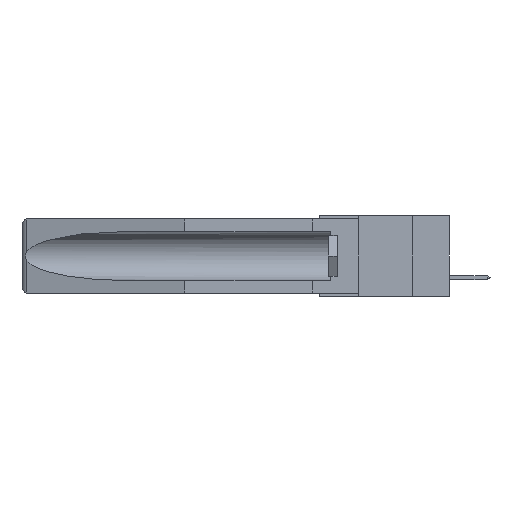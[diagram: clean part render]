
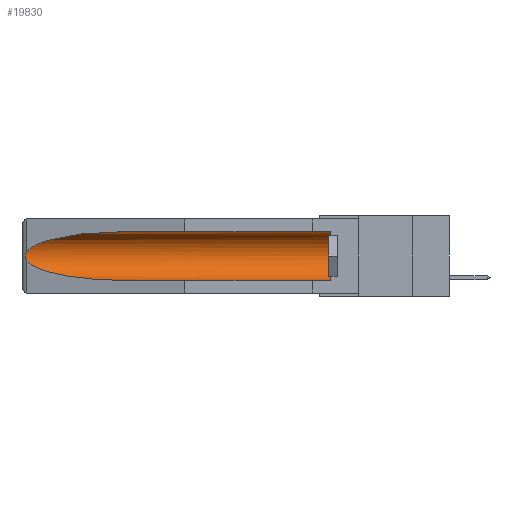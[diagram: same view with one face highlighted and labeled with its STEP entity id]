
A CAD part, left-side view. The second image highlights one B-rep face of the part: STEP entity #19830.
In plain terms, the highlighted cylindrical face has radius 2.857 mm (diameter 5.715 mm), a partial arc.
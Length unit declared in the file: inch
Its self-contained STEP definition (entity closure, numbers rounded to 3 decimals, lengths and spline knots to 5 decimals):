
#290 = EDGE_CURVE ( 'NONE', #24988, #15728, #14196, .T. ) ;
#362 = CARTESIAN_POINT ( 'NONE',  ( 0.155, 1.07973, -0.284 ) ) ;
#722 = ORIENTED_EDGE ( 'NONE', *, *, #5472, .T. ) ;
#1000 = ORIENTED_EDGE ( 'NONE', *, *, #20695, .T. ) ;
#1009 = CARTESIAN_POINT ( 'NONE',  ( 0.2675, 1.53308, -0.17534 ) ) ;
#1098 = CYLINDRICAL_SURFACE ( 'NONE', #19582, 0.1125 ) ;
#1209 = CARTESIAN_POINT ( 'NONE',  ( 0.26654, 1.53092, -0.15636 ) ) ;
#1514 = DIRECTION ( 'NONE',  ( 0., 1., 0. ) ) ;
#1770 = CARTESIAN_POINT ( 'NONE',  ( 0.25451, 1.48313, -0.09465 ) ) ;
#1946 = DIRECTION ( 'NONE',  ( 0., 0., 1. ) ) ;
#2255 = CARTESIAN_POINT ( 'NONE',  ( 0.25451, 1.48313, -0.24835 ) ) ;
#3594 = ORIENTED_EDGE ( 'NONE', *, *, #12901, .T. ) ;
#5472 = EDGE_CURVE ( 'NONE', #19635, #10450, #25865, .T. ) ;
#5909 = CARTESIAN_POINT ( 'NONE',  ( 0.2673, 1.53269, -0.17917 ) ) ;
#6745 = CARTESIAN_POINT ( 'NONE',  ( 0.26537, 1.52718, -0.19328 ) ) ;
#7039 = CARTESIAN_POINT ( 'NONE',  ( 0.26597, 1.5296, -0.19026 ) ) ;
#7882 = CARTESIAN_POINT ( 'NONE',  ( 0.155, 0.126, -0.1715 ) ) ;
#8403 = DIRECTION ( 'NONE',  ( 0., 0., 1. ) ) ;
#8800 = ORIENTED_EDGE ( 'NONE', *, *, #290, .T. ) ;
#8881 = VECTOR ( 'NONE', #13621, 39.37008 ) ;
#9677 = CARTESIAN_POINT ( 'NONE',  ( 0.21114, 1.30732, -0.284 ) ) ;
#10450 = VERTEX_POINT ( 'NONE', #31261 ) ;
#10668 = CARTESIAN_POINT ( 'NONE',  ( 0.2675, 1.53308, -0.16763 ) ) ;
#11177 = CARTESIAN_POINT ( 'NONE',  ( 0.155, -0.30754, -0.059 ) ) ;
#11340 = FACE_OUTER_BOUND ( 'NONE', #30940, .T. ) ;
#11903 = LINE ( 'NONE', #11177, #8881 ) ;
#12901 = EDGE_CURVE ( 'NONE', #15728, #19635, #11903, .T. ) ;
#13092 = CARTESIAN_POINT ( 'NONE',  ( 0.2673, 1.5327, -0.16383 ) ) ;
#13621 = DIRECTION ( 'NONE',  ( 0., 1., 0. ) ) ;
#13693 = ORIENTED_EDGE ( 'NONE', *, *, #15148, .F. ) ;
#13816 = B_SPLINE_CURVE_WITH_KNOTS ( 'NONE', 3,
 ( #25207, #15742, #1209, #13092, #10668, #1009, #5909, #31341, #7039, #6745 ),
 .UNSPECIFIED., .F., .F.,
 ( 4, 2, 2, 2, 4 ),
 ( 0., 0.00029, 0.00058, 0.00087, 0.00117 ),
 .UNSPECIFIED. ) ;
#13850 = CARTESIAN_POINT ( 'NONE',  ( 0.21114, 1.30732, -0.059 ) ) ;
#14196 = CIRCLE ( 'NONE', #25881, 0.1125 ) ;
#14233 = CARTESIAN_POINT ( 'NONE',  ( 0.155, -0.30754, -0.1715 ) ) ;
#14399 =( BOUNDED_CURVE ( )  B_SPLINE_CURVE ( 3, ( #31339, #2255, #9677, #31130 ),
 .UNSPECIFIED., .F., .F. ) 
 B_SPLINE_CURVE_WITH_KNOTS ( ( 4, 4 ),
 ( 0.1948, 1.5708 ),
 .UNSPECIFIED. ) 
 CURVE ( )  GEOMETRIC_REPRESENTATION_ITEM ( )  RATIONAL_B_SPLINE_CURVE ( ( 1., 0.848, 0.848, 1. ) ) 
 REPRESENTATION_ITEM ( '' )  );
#15148 = EDGE_CURVE ( 'NONE', #24988, #28561, #18654, .T. ) ;
#15728 = VERTEX_POINT ( 'NONE', #21690 ) ;
#15742 = CARTESIAN_POINT ( 'NONE',  ( 0.26597, 1.52961, -0.15275 ) ) ;
#18654 = LINE ( 'NONE', #23687, #25485 ) ;
#19528 = CARTESIAN_POINT ( 'NONE',  ( 0.155, 1.07973, -0.059 ) ) ;
#19582 = AXIS2_PLACEMENT_3D ( 'NONE', #14233, #26134, #1946 ) ;
#19635 = VERTEX_POINT ( 'NONE', #19528 ) ;
#19821 = EDGE_CURVE ( 'NONE', #10450, #24205, #13816, .T. ) ;
#19830 = ADVANCED_FACE ( 'NONE', ( #11340 ), #1098, .F. ) ;
#20695 = EDGE_CURVE ( 'NONE', #24205, #28561, #14399, .T. ) ;
#21100 = CARTESIAN_POINT ( 'NONE',  ( 0.155, 1.07973, -0.059 ) ) ;
#21198 = CARTESIAN_POINT ( 'NONE',  ( 0.26537, 1.52718, -0.14972 ) ) ;
#21690 = CARTESIAN_POINT ( 'NONE',  ( 0.155, 0.126, -0.059 ) ) ;
#22140 = CARTESIAN_POINT ( 'NONE',  ( 0.26537, 1.52718, -0.19328 ) ) ;
#23687 = CARTESIAN_POINT ( 'NONE',  ( 0.155, -0.30754, -0.284 ) ) ;
#24205 = VERTEX_POINT ( 'NONE', #22140 ) ;
#24988 = VERTEX_POINT ( 'NONE', #29843 ) ;
#25207 = CARTESIAN_POINT ( 'NONE',  ( 0.26537, 1.52718, -0.14972 ) ) ;
#25485 = VECTOR ( 'NONE', #1514, 39.37008 ) ;
#25599 = ORIENTED_EDGE ( 'NONE', *, *, #19821, .T. ) ;
#25865 =( BOUNDED_CURVE ( )  B_SPLINE_CURVE ( 3, ( #21100, #13850, #1770, #21198 ),
 .UNSPECIFIED., .F., .F. ) 
 B_SPLINE_CURVE_WITH_KNOTS ( ( 4, 4 ),
 ( 4.71239, 6.08839 ),
 .UNSPECIFIED. ) 
 CURVE ( )  GEOMETRIC_REPRESENTATION_ITEM ( )  RATIONAL_B_SPLINE_CURVE ( ( 1., 0.848, 0.848, 1. ) ) 
 REPRESENTATION_ITEM ( '' )  );
#25881 = AXIS2_PLACEMENT_3D ( 'NONE', #7882, #28140, #8403 ) ;
#26134 = DIRECTION ( 'NONE',  ( 0., 1., 0. ) ) ;
#28140 = DIRECTION ( 'NONE',  ( 0., -1., 0. ) ) ;
#28561 = VERTEX_POINT ( 'NONE', #362 ) ;
#29843 = CARTESIAN_POINT ( 'NONE',  ( 0.155, 0.126, -0.284 ) ) ;
#30940 = EDGE_LOOP ( 'NONE', ( #722, #25599, #1000, #13693, #8800, #3594 ) ) ;
#31130 = CARTESIAN_POINT ( 'NONE',  ( 0.155, 1.07973, -0.284 ) ) ;
#31261 = CARTESIAN_POINT ( 'NONE',  ( 0.26537, 1.52718, -0.14972 ) ) ;
#31339 = CARTESIAN_POINT ( 'NONE',  ( 0.26537, 1.52718, -0.19328 ) ) ;
#31341 = CARTESIAN_POINT ( 'NONE',  ( 0.26655, 1.53094, -0.18657 ) ) ;
